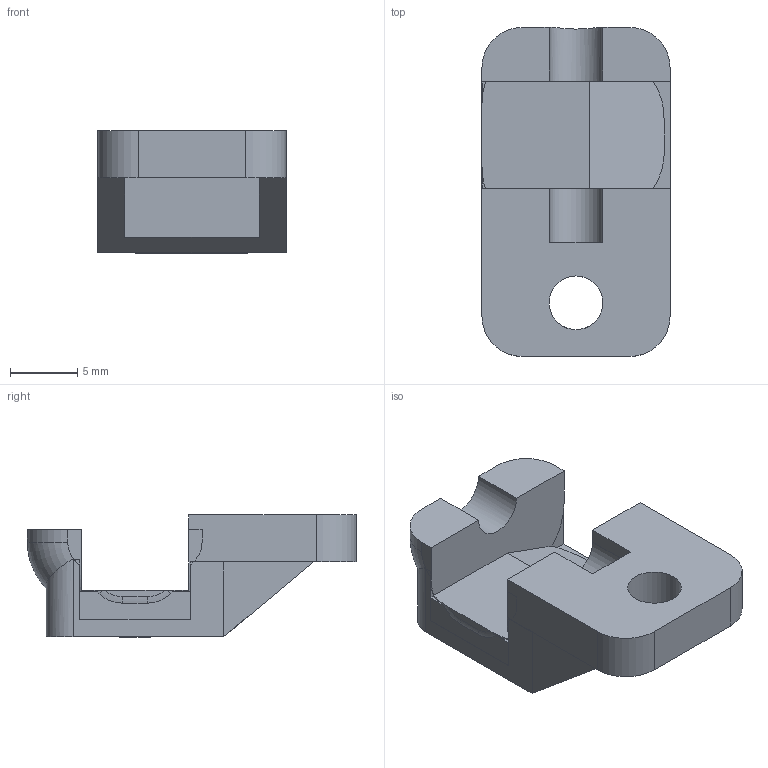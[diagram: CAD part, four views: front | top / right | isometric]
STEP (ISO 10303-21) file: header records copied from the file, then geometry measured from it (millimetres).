
FILE_DESCRIPTION(('FreeCAD Model'),'2;1');
FILE_NAME('gluty mag release retainer 2020.step','2020-04-04T17:48:47',('Author'),(''), 'Open CASCADE STEP processor 6.8','FreeCAD','Unknown');
FILE_SCHEMA(('AUTOMOTIVE_DESIGN_CC2 { 1 2 10303 214 -1 1 5 4 }'));
Length unit declared in the file: millimetre
Products named in the file (1): Pocket003
Bounding box: 14 x 24.5 x 9.1 mm (x, y, z)
Volume: 1503.1 mm3; surface area: 1478.5 mm2
Topology: 1 solids, 3 shells, 111 faces, 288 edges, 184 vertices
Faces by surface type: plane 75, cylinder 22, revolution 14
Full cylindrical faces by diameter (mm): 4 x1
Entity records: 16165 total; most frequent: CARTESIAN_POINT 10820, DIRECTION 842, ORIENTED_EDGE 576, PCURVE 576, DEFINITIONAL_REPRESENTATION 576, LINE 478, VECTOR 478, EDGE_CURVE 288
